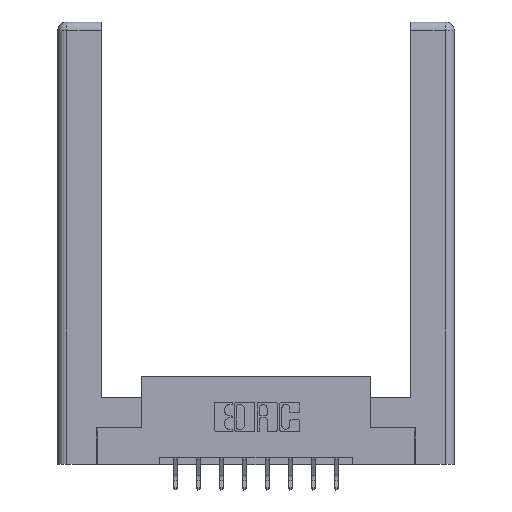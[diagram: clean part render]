
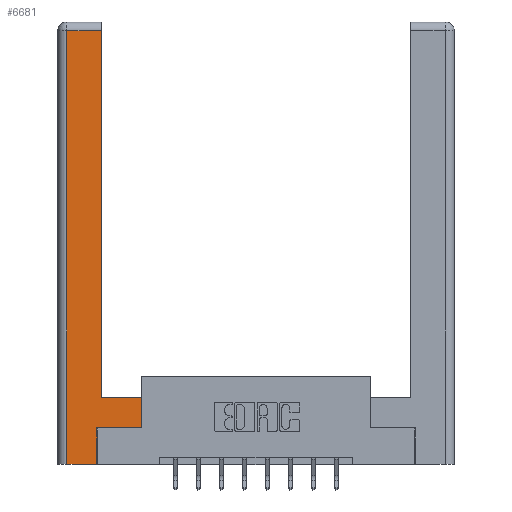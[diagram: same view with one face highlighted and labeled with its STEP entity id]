
A CAD part, top view. The second image highlights one B-rep face of the part: STEP entity #6681.
In plain terms, the highlighted planar face has unit normal (0, 0, 1).
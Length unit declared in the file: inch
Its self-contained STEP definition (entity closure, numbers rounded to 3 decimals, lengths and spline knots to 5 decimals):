
#9 = LINE ( 'NONE', #11351, #2481 ) ;
#144 = DIRECTION ( 'NONE',  ( 1., 0., 0. ) ) ;
#477 = ORIENTED_EDGE ( 'NONE', *, *, #701, .T. ) ;
#701 = EDGE_CURVE ( 'NONE', #4263, #6618, #11815, .T. ) ;
#872 = DIRECTION ( 'NONE',  ( 0., 1., 0. ) ) ;
#906 = CARTESIAN_POINT ( 'NONE',  ( 0.565, 0.45, 0. ) ) ;
#1049 = VERTEX_POINT ( 'NONE', #4886 ) ;
#1558 = DIRECTION ( 'NONE',  ( 0., 0., -1. ) ) ;
#1777 = DIRECTION ( 'NONE',  ( 0., -1., 0. ) ) ;
#1796 = LINE ( 'NONE', #9915, #12506 ) ;
#1877 = EDGE_CURVE ( 'NONE', #12969, #1049, #3156, .T. ) ;
#2263 = ORIENTED_EDGE ( 'NONE', *, *, #9864, .T. ) ;
#2481 = VECTOR ( 'NONE', #7116, 39.37008 ) ;
#2534 = ORIENTED_EDGE ( 'NONE', *, *, #3982, .T. ) ;
#2587 = PLANE ( 'NONE',  #5795 ) ;
#2666 = DIRECTION ( 'NONE',  ( -1., 0., 0. ) ) ;
#2690 = EDGE_CURVE ( 'NONE', #6618, #5780, #9930, .T. ) ;
#2715 = EDGE_CURVE ( 'NONE', #10265, #12969, #9, .T. ) ;
#2917 = CARTESIAN_POINT ( 'NONE',  ( 0.295, 3., 0. ) ) ;
#3046 = CARTESIAN_POINT ( 'NONE',  ( 0.265, 0., 0. ) ) ;
#3156 = LINE ( 'NONE', #2917, #5888 ) ;
#3445 = DIRECTION ( 'NONE',  ( 0., 1., 0. ) ) ;
#3982 = EDGE_CURVE ( 'NONE', #5780, #12155, #6998, .T. ) ;
#3983 = FACE_OUTER_BOUND ( 'NONE', #9851, .T. ) ;
#4263 = VERTEX_POINT ( 'NONE', #7032 ) ;
#4529 = EDGE_CURVE ( 'NONE', #12155, #10265, #13316, .T. ) ;
#4886 = CARTESIAN_POINT ( 'NONE',  ( 0.295, 2.94, 0. ) ) ;
#4993 = ORIENTED_EDGE ( 'NONE', *, *, #2715, .T. ) ;
#5101 = DIRECTION ( 'NONE',  ( 0., 1., 0. ) ) ;
#5131 = CARTESIAN_POINT ( 'NONE',  ( 0.565, 0.245, 0. ) ) ;
#5285 = VECTOR ( 'NONE', #144, 39.37008 ) ;
#5780 = VERTEX_POINT ( 'NONE', #11945 ) ;
#5795 = AXIS2_PLACEMENT_3D ( 'NONE', #8695, #1558, #2666 ) ;
#5836 = ORIENTED_EDGE ( 'NONE', *, *, #9552, .T. ) ;
#5888 = VECTOR ( 'NONE', #872, 39.37008 ) ;
#6111 = VERTEX_POINT ( 'NONE', #6936 ) ;
#6311 = DIRECTION ( 'NONE',  ( 1., 0., 0. ) ) ;
#6618 = VERTEX_POINT ( 'NONE', #3046 ) ;
#6681 = ADVANCED_FACE ( 'NONE', ( #3983 ), #2587, .F. ) ;
#6936 = CARTESIAN_POINT ( 'NONE',  ( 0.0615, 2.94, 0. ) ) ;
#6998 = LINE ( 'NONE', #5131, #12862 ) ;
#7032 = CARTESIAN_POINT ( 'NONE',  ( 0.0615, 0., 0. ) ) ;
#7116 = DIRECTION ( 'NONE',  ( -1., 0., 0. ) ) ;
#7172 = VECTOR ( 'NONE', #5101, 39.37008 ) ;
#7323 = CARTESIAN_POINT ( 'NONE',  ( 0.0615, 2.94, 0. ) ) ;
#8519 = ORIENTED_EDGE ( 'NONE', *, *, #1877, .T. ) ;
#8695 = CARTESIAN_POINT ( 'NONE',  ( 0., 0., 0. ) ) ;
#9552 = EDGE_CURVE ( 'NONE', #6111, #4263, #1796, .T. ) ;
#9851 = EDGE_LOOP ( 'NONE', ( #8519, #2263, #5836, #477, #13450, #2534, #11592, #4993 ) ) ;
#9864 = EDGE_CURVE ( 'NONE', #1049, #6111, #13308, .T. ) ;
#9915 = CARTESIAN_POINT ( 'NONE',  ( 0.0615, 0., 0. ) ) ;
#9930 = LINE ( 'NONE', #12431, #7172 ) ;
#10265 = VERTEX_POINT ( 'NONE', #906 ) ;
#10680 = CARTESIAN_POINT ( 'NONE',  ( 0.295, 0.45, 0. ) ) ;
#11351 = CARTESIAN_POINT ( 'NONE',  ( 0.295, 0.45, 0. ) ) ;
#11592 = ORIENTED_EDGE ( 'NONE', *, *, #4529, .T. ) ;
#11693 = VECTOR ( 'NONE', #12652, 39.37008 ) ;
#11815 = LINE ( 'NONE', #12604, #5285 ) ;
#11945 = CARTESIAN_POINT ( 'NONE',  ( 0.265, 0.245, 0. ) ) ;
#12155 = VERTEX_POINT ( 'NONE', #12246 ) ;
#12246 = CARTESIAN_POINT ( 'NONE',  ( 0.565, 0.245, 0. ) ) ;
#12431 = CARTESIAN_POINT ( 'NONE',  ( 0.265, 0.245, 0. ) ) ;
#12506 = VECTOR ( 'NONE', #1777, 39.37008 ) ;
#12604 = CARTESIAN_POINT ( 'NONE',  ( 0.265, 0., 0. ) ) ;
#12652 = DIRECTION ( 'NONE',  ( -1., 0., 0. ) ) ;
#12675 = VECTOR ( 'NONE', #3445, 39.37008 ) ;
#12846 = CARTESIAN_POINT ( 'NONE',  ( 0.565, 0.45, 0. ) ) ;
#12862 = VECTOR ( 'NONE', #6311, 39.37008 ) ;
#12969 = VERTEX_POINT ( 'NONE', #10680 ) ;
#13308 = LINE ( 'NONE', #7323, #11693 ) ;
#13316 = LINE ( 'NONE', #12846, #12675 ) ;
#13450 = ORIENTED_EDGE ( 'NONE', *, *, #2690, .T. ) ;
